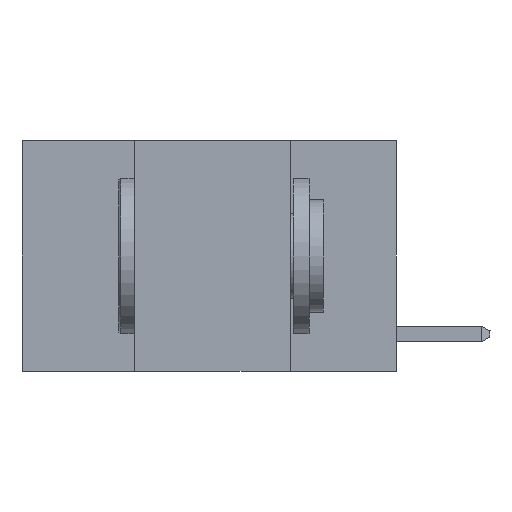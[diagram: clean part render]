
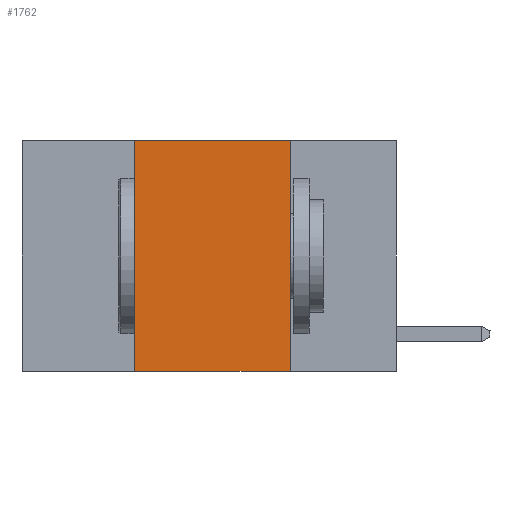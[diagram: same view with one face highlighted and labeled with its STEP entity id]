
A CAD part, left-side view. The second image highlights one B-rep face of the part: STEP entity #1762.
In plain terms, the highlighted planar face has unit normal (-1, 0, 0).
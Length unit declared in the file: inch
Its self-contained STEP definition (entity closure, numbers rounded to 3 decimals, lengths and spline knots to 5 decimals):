
#509 = CARTESIAN_POINT ( 'NONE',  ( 0., 0.42, -0.37 ) ) ;
#800 = EDGE_CURVE ( 'NONE', #8035, #29979, #17227, .T. ) ;
#1762 = ADVANCED_FACE ( 'NONE', ( #9476 ), #4766, .F. ) ;
#2416 = VERTEX_POINT ( 'NONE', #29318 ) ;
#2688 = DIRECTION ( 'NONE',  ( 0., -1., 0. ) ) ;
#2702 = ORIENTED_EDGE ( 'NONE', *, *, #6826, .F. ) ;
#4416 = ORIENTED_EDGE ( 'NONE', *, *, #17305, .F. ) ;
#4587 = VECTOR ( 'NONE', #7145, 39.37008 ) ;
#4766 = PLANE ( 'NONE',  #9154 ) ;
#6826 = EDGE_CURVE ( 'NONE', #2416, #29979, #7502, .T. ) ;
#7145 = DIRECTION ( 'NONE',  ( 0., -1., 0. ) ) ;
#7502 = LINE ( 'NONE', #16854, #25324 ) ;
#8035 = VERTEX_POINT ( 'NONE', #509 ) ;
#9154 = AXIS2_PLACEMENT_3D ( 'NONE', #16114, #16558, #13477 ) ;
#9291 = CARTESIAN_POINT ( 'NONE',  ( 0., 0.6, 0. ) ) ;
#9476 = FACE_OUTER_BOUND ( 'NONE', #28353, .T. ) ;
#13477 = DIRECTION ( 'NONE',  ( 0., 0., -1. ) ) ;
#13630 = CARTESIAN_POINT ( 'NONE',  ( 0., 0.42, 0. ) ) ;
#14699 = DIRECTION ( 'NONE',  ( 0., 0., -1. ) ) ;
#16114 = CARTESIAN_POINT ( 'NONE',  ( 0., 0.6, 0. ) ) ;
#16558 = DIRECTION ( 'NONE',  ( 1., 0., 0. ) ) ;
#16854 = CARTESIAN_POINT ( 'NONE',  ( 0., 0.17, 0. ) ) ;
#16922 = CARTESIAN_POINT ( 'NONE',  ( 0., 0.6, -0.37 ) ) ;
#17227 = LINE ( 'NONE', #16922, #17927 ) ;
#17305 = EDGE_CURVE ( 'NONE', #17656, #2416, #23384, .T. ) ;
#17632 = CARTESIAN_POINT ( 'NONE',  ( 0., 0.42, 0. ) ) ;
#17656 = VERTEX_POINT ( 'NONE', #13630 ) ;
#17927 = VECTOR ( 'NONE', #2688, 39.37008 ) ;
#17958 = ORIENTED_EDGE ( 'NONE', *, *, #24429, .F. ) ;
#20375 = LINE ( 'NONE', #17632, #29231 ) ;
#20638 = ORIENTED_EDGE ( 'NONE', *, *, #800, .T. ) ;
#23384 = LINE ( 'NONE', #9291, #4587 ) ;
#24429 = EDGE_CURVE ( 'NONE', #8035, #17656, #20375, .T. ) ;
#25324 = VECTOR ( 'NONE', #14699, 39.37008 ) ;
#27362 = CARTESIAN_POINT ( 'NONE',  ( 0., 0.17, -0.37 ) ) ;
#28353 = EDGE_LOOP ( 'NONE', ( #2702, #4416, #17958, #20638 ) ) ;
#29231 = VECTOR ( 'NONE', #29685, 39.37008 ) ;
#29318 = CARTESIAN_POINT ( 'NONE',  ( 0., 0.17, 0. ) ) ;
#29685 = DIRECTION ( 'NONE',  ( 0., 0., 1. ) ) ;
#29979 = VERTEX_POINT ( 'NONE', #27362 ) ;
